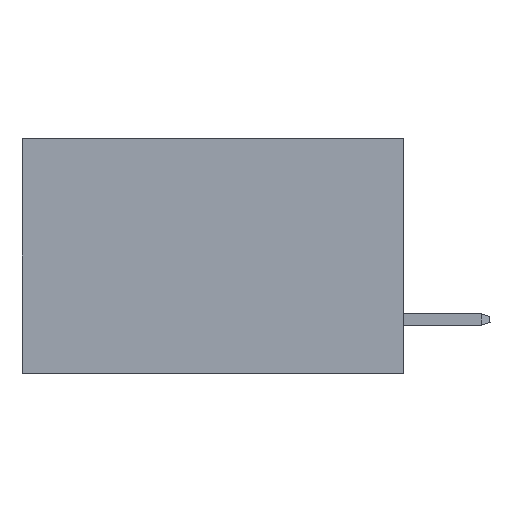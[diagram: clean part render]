
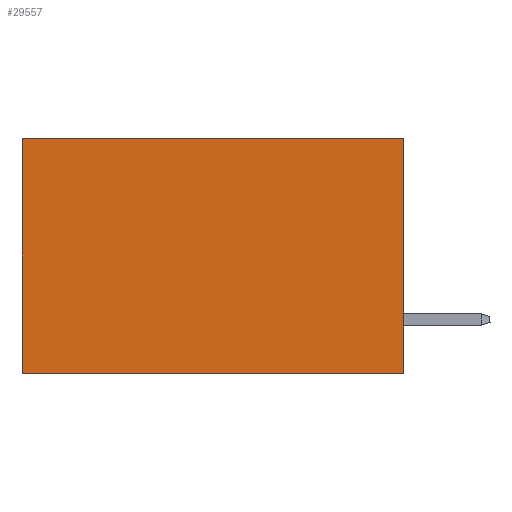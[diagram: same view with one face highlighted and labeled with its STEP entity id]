
A CAD part, left-side view. The second image highlights one B-rep face of the part: STEP entity #29557.
In plain terms, the highlighted planar face has unit normal (-1, 0, 0).
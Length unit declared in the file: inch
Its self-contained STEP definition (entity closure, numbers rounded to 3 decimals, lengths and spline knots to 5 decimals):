
#82 = EDGE_CURVE ( 'NONE', #26893, #6404, #16814, .T. ) ;
#270 = DIRECTION ( 'NONE',  ( 0., 0., -1. ) ) ;
#470 = CARTESIAN_POINT ( 'NONE',  ( 0.2875, 0., 0. ) ) ;
#2794 = ORIENTED_EDGE ( 'NONE', *, *, #24491, .T. ) ;
#4451 = CARTESIAN_POINT ( 'NONE',  ( 0.2875, 0.6, -0.37 ) ) ;
#4649 = CARTESIAN_POINT ( 'NONE',  ( 0.2875, 0., 0. ) ) ;
#5592 = EDGE_LOOP ( 'NONE', ( #2794, #36950, #16552, #12150 ) ) ;
#6404 = VERTEX_POINT ( 'NONE', #9201 ) ;
#6573 = VECTOR ( 'NONE', #20015, 39.37008 ) ;
#7453 = CARTESIAN_POINT ( 'NONE',  ( 0.2875, 0., -0.37 ) ) ;
#7506 = FACE_OUTER_BOUND ( 'NONE', #5592, .T. ) ;
#8219 = LINE ( 'NONE', #34969, #25695 ) ;
#9201 = CARTESIAN_POINT ( 'NONE',  ( 0.2875, 0.6, 0. ) ) ;
#12150 = ORIENTED_EDGE ( 'NONE', *, *, #82, .T. ) ;
#13501 = VECTOR ( 'NONE', #270, 39.37008 ) ;
#16176 = VERTEX_POINT ( 'NONE', #4451 ) ;
#16459 = AXIS2_PLACEMENT_3D ( 'NONE', #19687, #31864, #35038 ) ;
#16552 = ORIENTED_EDGE ( 'NONE', *, *, #35642, .F. ) ;
#16814 = LINE ( 'NONE', #22979, #6573 ) ;
#19687 = CARTESIAN_POINT ( 'NONE',  ( 0.2875, 0., 0. ) ) ;
#20015 = DIRECTION ( 'NONE',  ( 0., 1., 0. ) ) ;
#22667 = VERTEX_POINT ( 'NONE', #7453 ) ;
#22856 = PLANE ( 'NONE',  #16459 ) ;
#22979 = CARTESIAN_POINT ( 'NONE',  ( 0.2875, 0., 0. ) ) ;
#23567 = DIRECTION ( 'NONE',  ( 0., 0., -1. ) ) ;
#24491 = EDGE_CURVE ( 'NONE', #6404, #16176, #39144, .T. ) ;
#25695 = VECTOR ( 'NONE', #32178, 39.37008 ) ;
#26893 = VERTEX_POINT ( 'NONE', #4649 ) ;
#27203 = VECTOR ( 'NONE', #23567, 39.37008 ) ;
#29557 = ADVANCED_FACE ( 'NONE', ( #7506 ), #22856, .F. ) ;
#31864 = DIRECTION ( 'NONE',  ( 1., 0., 0. ) ) ;
#32178 = DIRECTION ( 'NONE',  ( 0., 1., 0. ) ) ;
#33343 = CARTESIAN_POINT ( 'NONE',  ( 0.2875, 0.6, 0. ) ) ;
#34969 = CARTESIAN_POINT ( 'NONE',  ( 0.2875, 0., -0.37 ) ) ;
#35038 = DIRECTION ( 'NONE',  ( 0., 0., -1. ) ) ;
#35642 = EDGE_CURVE ( 'NONE', #26893, #22667, #36779, .T. ) ;
#36779 = LINE ( 'NONE', #470, #13501 ) ;
#36950 = ORIENTED_EDGE ( 'NONE', *, *, #38547, .F. ) ;
#38547 = EDGE_CURVE ( 'NONE', #22667, #16176, #8219, .T. ) ;
#39144 = LINE ( 'NONE', #33343, #27203 ) ;
